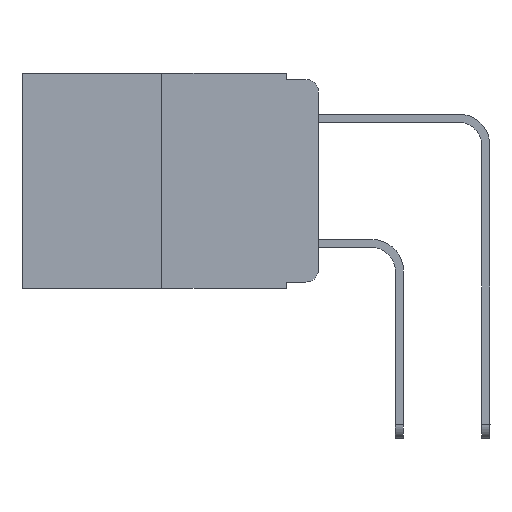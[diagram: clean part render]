
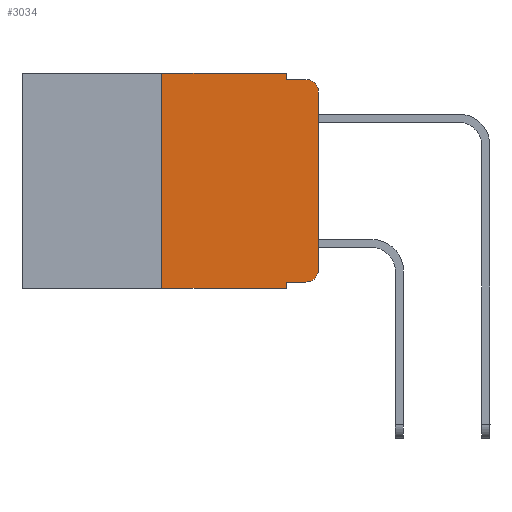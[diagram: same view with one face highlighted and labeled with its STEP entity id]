
A CAD part, left-side view. The second image highlights one B-rep face of the part: STEP entity #3034.
In plain terms, the highlighted planar face has unit normal (-1, 0, 0).
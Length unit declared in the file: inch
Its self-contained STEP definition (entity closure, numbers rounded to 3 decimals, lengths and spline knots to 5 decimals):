
#411 = VECTOR ( 'NONE', #18185, 39.37008 ) ;
#607 = DIRECTION ( 'NONE',  ( 0., -1., 0. ) ) ;
#756 = DIRECTION ( 'NONE',  ( 0., 0., 1. ) ) ;
#1160 = VECTOR ( 'NONE', #18131, 39.37008 ) ;
#1260 = EDGE_LOOP ( 'NONE', ( #9794, #16360, #5596, #2994, #12315, #15967, #7516, #7046, #2481, #11140 ) ) ;
#1466 = DIRECTION ( 'NONE',  ( 0., 0., -1. ) ) ;
#1583 = CARTESIAN_POINT ( 'NONE',  ( 0., 0.02, -0.03 ) ) ;
#1652 = VECTOR ( 'NONE', #4674, 39.37008 ) ;
#2080 = EDGE_CURVE ( 'NONE', #7670, #14446, #14702, .T. ) ;
#2393 = VECTOR ( 'NONE', #13278, 39.37008 ) ;
#2481 = ORIENTED_EDGE ( 'NONE', *, *, #2080, .T. ) ;
#2583 = VERTEX_POINT ( 'NONE', #11265 ) ;
#2636 = CARTESIAN_POINT ( 'NONE',  ( 0., 0.02, -0.313 ) ) ;
#2994 = ORIENTED_EDGE ( 'NONE', *, *, #10751, .F. ) ;
#3011 = EDGE_CURVE ( 'NONE', #16118, #15656, #13086, .T. ) ;
#3034 = ADVANCED_FACE ( 'NONE', ( #3130 ), #9801, .F. ) ;
#3130 = FACE_OUTER_BOUND ( 'NONE', #1260, .T. ) ;
#3665 = VERTEX_POINT ( 'NONE', #15799 ) ;
#4184 = DIRECTION ( 'NONE',  ( -1., 0., 0. ) ) ;
#4674 = DIRECTION ( 'NONE',  ( 0., 0., -1. ) ) ;
#4874 = VECTOR ( 'NONE', #607, 39.37008 ) ;
#5596 = ORIENTED_EDGE ( 'NONE', *, *, #20183, .F. ) ;
#6643 = DIRECTION ( 'NONE',  ( -1., 0., 0. ) ) ;
#7046 = ORIENTED_EDGE ( 'NONE', *, *, #18621, .F. ) ;
#7049 = AXIS2_PLACEMENT_3D ( 'NONE', #2636, #4184, #19082 ) ;
#7516 = ORIENTED_EDGE ( 'NONE', *, *, #3011, .T. ) ;
#7670 = VERTEX_POINT ( 'NONE', #21514 ) ;
#7694 = VERTEX_POINT ( 'NONE', #18579 ) ;
#8312 = EDGE_CURVE ( 'NONE', #14446, #10841, #17566, .T. ) ;
#8817 = EDGE_CURVE ( 'NONE', #10841, #17739, #18948, .T. ) ;
#9411 = CIRCLE ( 'NONE', #21606, 0.02 ) ;
#9594 = DIRECTION ( 'NONE',  ( 0., 0., -1. ) ) ;
#9794 = ORIENTED_EDGE ( 'NONE', *, *, #8817, .T. ) ;
#9801 = PLANE ( 'NONE',  #14815 ) ;
#10212 = CARTESIAN_POINT ( 'NONE',  ( 0., 0.473, 0. ) ) ;
#10240 = EDGE_CURVE ( 'NONE', #16118, #2583, #20912, .T. ) ;
#10682 = LINE ( 'NONE', #17511, #4874 ) ;
#10749 = CARTESIAN_POINT ( 'NONE',  ( 0., 0.051, -0.343 ) ) ;
#10751 = EDGE_CURVE ( 'NONE', #19356, #7694, #12987, .T. ) ;
#10841 = VERTEX_POINT ( 'NONE', #18349 ) ;
#11140 = ORIENTED_EDGE ( 'NONE', *, *, #8312, .T. ) ;
#11188 = CARTESIAN_POINT ( 'NONE',  ( 0., 0.051, -0.333 ) ) ;
#11265 = CARTESIAN_POINT ( 'NONE',  ( 0., 0.25, 0. ) ) ;
#12315 = ORIENTED_EDGE ( 'NONE', *, *, #20498, .F. ) ;
#12987 = LINE ( 'NONE', #17941, #17921 ) ;
#13041 = CARTESIAN_POINT ( 'NONE',  ( 0., 0., -0.03 ) ) ;
#13086 = LINE ( 'NONE', #21287, #1160 ) ;
#13278 = DIRECTION ( 'NONE',  ( 0., -1., 0. ) ) ;
#14363 = CARTESIAN_POINT ( 'NONE',  ( 0., 0.02, -0.333 ) ) ;
#14446 = VERTEX_POINT ( 'NONE', #14363 ) ;
#14550 = DIRECTION ( 'NONE',  ( 0., 0., -1. ) ) ;
#14702 = LINE ( 'NONE', #11188, #411 ) ;
#14815 = AXIS2_PLACEMENT_3D ( 'NONE', #16521, #17933, #1466 ) ;
#15656 = VERTEX_POINT ( 'NONE', #10749 ) ;
#15796 = CARTESIAN_POINT ( 'NONE',  ( 0., 0., 0. ) ) ;
#15799 = CARTESIAN_POINT ( 'NONE',  ( 0., 0.02, -0.01 ) ) ;
#15967 = ORIENTED_EDGE ( 'NONE', *, *, #10240, .F. ) ;
#16023 = CARTESIAN_POINT ( 'NONE',  ( 0., 0.051, 0. ) ) ;
#16118 = VERTEX_POINT ( 'NONE', #20781 ) ;
#16152 = CARTESIAN_POINT ( 'NONE',  ( 0., 0.25, 0. ) ) ;
#16360 = ORIENTED_EDGE ( 'NONE', *, *, #21142, .T. ) ;
#16521 = CARTESIAN_POINT ( 'NONE',  ( 0., 0.473, 0. ) ) ;
#17049 = LINE ( 'NONE', #10212, #2393 ) ;
#17511 = CARTESIAN_POINT ( 'NONE',  ( 0., 0.051, -0.01 ) ) ;
#17566 = CIRCLE ( 'NONE', #7049, 0.02 ) ;
#17723 = VECTOR ( 'NONE', #756, 39.37008 ) ;
#17739 = VERTEX_POINT ( 'NONE', #13041 ) ;
#17921 = VECTOR ( 'NONE', #9594, 39.37008 ) ;
#17933 = DIRECTION ( 'NONE',  ( 1., 0., 0. ) ) ;
#17941 = CARTESIAN_POINT ( 'NONE',  ( 0., 0.051, 0. ) ) ;
#17943 = CARTESIAN_POINT ( 'NONE',  ( 0., 0.051, 0. ) ) ;
#18131 = DIRECTION ( 'NONE',  ( 0., -1., 0. ) ) ;
#18185 = DIRECTION ( 'NONE',  ( 0., -1., 0. ) ) ;
#18349 = CARTESIAN_POINT ( 'NONE',  ( 0., 0., -0.313 ) ) ;
#18579 = CARTESIAN_POINT ( 'NONE',  ( 0., 0.051, -0.01 ) ) ;
#18621 = EDGE_CURVE ( 'NONE', #7670, #15656, #21083, .T. ) ;
#18948 = LINE ( 'NONE', #15796, #17723 ) ;
#19082 = DIRECTION ( 'NONE',  ( 0., 0., -1. ) ) ;
#19197 = DIRECTION ( 'NONE',  ( 0., 0., 1. ) ) ;
#19297 = VECTOR ( 'NONE', #19197, 39.37008 ) ;
#19356 = VERTEX_POINT ( 'NONE', #16023 ) ;
#20183 = EDGE_CURVE ( 'NONE', #7694, #3665, #10682, .T. ) ;
#20498 = EDGE_CURVE ( 'NONE', #2583, #19356, #17049, .T. ) ;
#20781 = CARTESIAN_POINT ( 'NONE',  ( 0., 0.25, -0.343 ) ) ;
#20912 = LINE ( 'NONE', #16152, #19297 ) ;
#21083 = LINE ( 'NONE', #17943, #1652 ) ;
#21142 = EDGE_CURVE ( 'NONE', #17739, #3665, #9411, .T. ) ;
#21287 = CARTESIAN_POINT ( 'NONE',  ( 0., 0.473, -0.343 ) ) ;
#21514 = CARTESIAN_POINT ( 'NONE',  ( 0., 0.051, -0.333 ) ) ;
#21606 = AXIS2_PLACEMENT_3D ( 'NONE', #1583, #6643, #14550 ) ;
